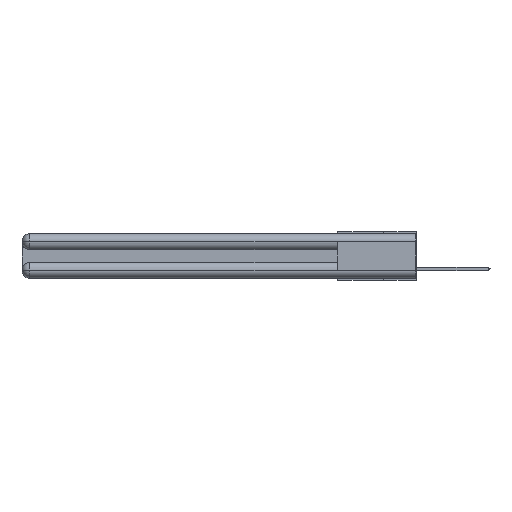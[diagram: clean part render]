
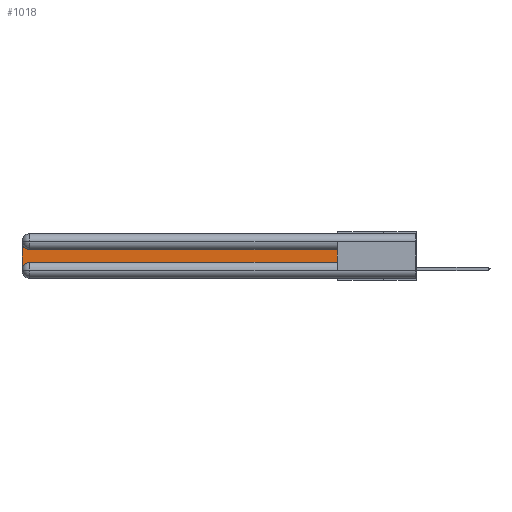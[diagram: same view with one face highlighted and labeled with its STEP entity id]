
A CAD part, left-side view. The second image highlights one B-rep face of the part: STEP entity #1018.
In plain terms, the highlighted planar face has unit normal (-1, 0, 0).
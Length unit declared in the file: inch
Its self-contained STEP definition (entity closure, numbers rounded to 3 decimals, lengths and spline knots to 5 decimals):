
#1018 = ADVANCED_FACE ( 'NONE', ( #17464 ), #11689, .F. ) ;
#1499 = VERTEX_POINT ( 'NONE', #21849 ) ;
#2106 = CARTESIAN_POINT ( 'NONE',  ( 0.075, 2.94, -0.0625 ) ) ;
#2223 = EDGE_CURVE ( 'NONE', #4001, #19249, #20361, .T. ) ;
#2287 = DIRECTION ( 'NONE',  ( 0., 0., -1. ) ) ;
#2601 = ORIENTED_EDGE ( 'NONE', *, *, #2223, .T. ) ;
#2902 = VERTEX_POINT ( 'NONE', #6576 ) ;
#3198 = AXIS2_PLACEMENT_3D ( 'NONE', #21509, #25850, #13027 ) ;
#3251 = ORIENTED_EDGE ( 'NONE', *, *, #22790, .T. ) ;
#3340 = VECTOR ( 'NONE', #6382, 39.37008 ) ;
#3890 = CARTESIAN_POINT ( 'NONE',  ( 0.075, 0.6, -0.2175 ) ) ;
#4001 = VERTEX_POINT ( 'NONE', #7360 ) ;
#4026 = LINE ( 'NONE', #16473, #3340 ) ;
#5002 = DIRECTION ( 'NONE',  ( 0., 1., 0. ) ) ;
#6382 = DIRECTION ( 'NONE',  ( 0., 0., -1. ) ) ;
#6424 = ORIENTED_EDGE ( 'NONE', *, *, #24968, .T. ) ;
#6576 = CARTESIAN_POINT ( 'NONE',  ( 0.075, 0.6, -0.1225 ) ) ;
#7140 = CIRCLE ( 'NONE', #15864, 0.06 ) ;
#7360 = CARTESIAN_POINT ( 'NONE',  ( 0.075, 2.94, -0.2175 ) ) ;
#8575 = DIRECTION ( 'NONE',  ( 1., 0., 0. ) ) ;
#8972 = ORIENTED_EDGE ( 'NONE', *, *, #10252, .T. ) ;
#10121 = EDGE_LOOP ( 'NONE', ( #8972, #3251, #6424, #19085, #2601, #12103 ) ) ;
#10252 = EDGE_CURVE ( 'NONE', #2902, #16829, #10645, .T. ) ;
#10645 = LINE ( 'NONE', #24100, #20000 ) ;
#11689 = PLANE ( 'NONE',  #12794 ) ;
#12103 = ORIENTED_EDGE ( 'NONE', *, *, #16269, .T. ) ;
#12468 = CARTESIAN_POINT ( 'NONE',  ( 0.075, 3., -0.2775 ) ) ;
#12794 = AXIS2_PLACEMENT_3D ( 'NONE', #26819, #22312, #13820 ) ;
#13027 = DIRECTION ( 'NONE',  ( 0., 0., -1. ) ) ;
#13157 = CARTESIAN_POINT ( 'NONE',  ( 0.075, 2.94, -0.1225 ) ) ;
#13209 = CARTESIAN_POINT ( 'NONE',  ( 0.075, 0.6, -0.2175 ) ) ;
#13820 = DIRECTION ( 'NONE',  ( 0., 0., -1. ) ) ;
#14536 = DIRECTION ( 'NONE',  ( 0., 0., 1. ) ) ;
#15864 = AXIS2_PLACEMENT_3D ( 'NONE', #2106, #8575, #2287 ) ;
#16146 = CARTESIAN_POINT ( 'NONE',  ( 0.075, 0.6, -0.2175 ) ) ;
#16269 = EDGE_CURVE ( 'NONE', #19249, #2902, #17869, .T. ) ;
#16473 = CARTESIAN_POINT ( 'NONE',  ( 0.075, 3., -0.2175 ) ) ;
#16829 = VERTEX_POINT ( 'NONE', #13157 ) ;
#17156 = DIRECTION ( 'NONE',  ( 0., -1., 0. ) ) ;
#17464 = FACE_OUTER_BOUND ( 'NONE', #10121, .T. ) ;
#17869 = LINE ( 'NONE', #3890, #21163 ) ;
#19085 = ORIENTED_EDGE ( 'NONE', *, *, #20524, .T. ) ;
#19249 = VERTEX_POINT ( 'NONE', #16146 ) ;
#20000 = VECTOR ( 'NONE', #5002, 39.37008 ) ;
#20361 = LINE ( 'NONE', #13209, #26412 ) ;
#20524 = EDGE_CURVE ( 'NONE', #23220, #4001, #25687, .T. ) ;
#21163 = VECTOR ( 'NONE', #14536, 39.37008 ) ;
#21509 = CARTESIAN_POINT ( 'NONE',  ( 0.075, 2.94, -0.2775 ) ) ;
#21849 = CARTESIAN_POINT ( 'NONE',  ( 0.075, 3., -0.0625 ) ) ;
#22312 = DIRECTION ( 'NONE',  ( 1., 0., 0. ) ) ;
#22790 = EDGE_CURVE ( 'NONE', #16829, #1499, #7140, .T. ) ;
#23220 = VERTEX_POINT ( 'NONE', #12468 ) ;
#24100 = CARTESIAN_POINT ( 'NONE',  ( 0.075, 0.6, -0.1225 ) ) ;
#24968 = EDGE_CURVE ( 'NONE', #1499, #23220, #4026, .T. ) ;
#25687 = CIRCLE ( 'NONE', #3198, 0.06 ) ;
#25850 = DIRECTION ( 'NONE',  ( 1., 0., 0. ) ) ;
#26412 = VECTOR ( 'NONE', #17156, 39.37008 ) ;
#26819 = CARTESIAN_POINT ( 'NONE',  ( 0.075, 3., -0.1225 ) ) ;
